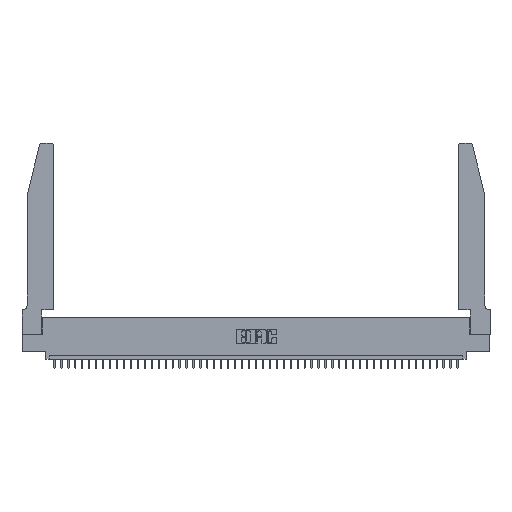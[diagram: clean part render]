
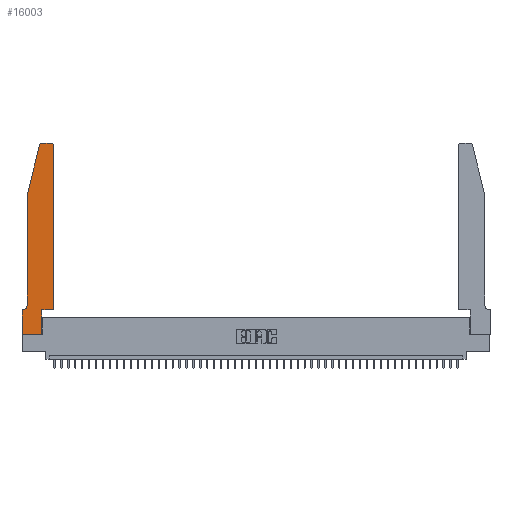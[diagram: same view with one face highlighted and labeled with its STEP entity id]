
A CAD part, top view. The second image highlights one B-rep face of the part: STEP entity #16003.
In plain terms, the highlighted planar face has unit normal (0, 0, 1).
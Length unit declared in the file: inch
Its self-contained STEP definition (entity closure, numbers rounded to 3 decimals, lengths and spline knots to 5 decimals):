
#1456 = AXIS2_PLACEMENT_3D ( 'NONE', #13694, #27518, #30842 ) ;
#2073 = VECTOR ( 'NONE', #4219, 39.37008 ) ;
#2291 = VERTEX_POINT ( 'NONE', #4777 ) ;
#2474 = ORIENTED_EDGE ( 'NONE', *, *, #27144, .T. ) ;
#3057 = CIRCLE ( 'NONE', #18257, 0.07 ) ;
#3388 = LINE ( 'NONE', #43634, #18350 ) ;
#4219 = DIRECTION ( 'NONE',  ( 0., 1., 0. ) ) ;
#4227 = CARTESIAN_POINT ( 'NONE',  ( 0., 0., 0.37 ) ) ;
#4251 = EDGE_CURVE ( 'NONE', #35111, #40724, #8358, .T. ) ;
#4667 = ORIENTED_EDGE ( 'NONE', *, *, #15329, .T. ) ;
#4777 = CARTESIAN_POINT ( 'NONE',  ( 0.0055, 0.35, 0.37 ) ) ;
#4821 = CIRCLE ( 'NONE', #31468, 0.03 ) ;
#4933 = LINE ( 'NONE', #8534, #8687 ) ;
#6106 = VECTOR ( 'NONE', #23300, 39.37008 ) ;
#6298 = PLANE ( 'NONE',  #1456 ) ;
#6853 = EDGE_CURVE ( 'NONE', #2291, #31830, #31171, .T. ) ;
#6995 = ORIENTED_EDGE ( 'NONE', *, *, #8389, .T. ) ;
#7415 = DIRECTION ( 'NONE',  ( 0., 1., 0. ) ) ;
#8043 = DIRECTION ( 'NONE',  ( -0.239, -0.971, 0. ) ) ;
#8358 = CIRCLE ( 'NONE', #34991, 0.03 ) ;
#8389 = EDGE_CURVE ( 'NONE', #27132, #35111, #39346, .T. ) ;
#8534 = CARTESIAN_POINT ( 'NONE',  ( 0.0755, 2., 0.37 ) ) ;
#8687 = VECTOR ( 'NONE', #8043, 39.37008 ) ;
#8797 = DIRECTION ( 'NONE',  ( -1., 0., 0. ) ) ;
#11934 = CARTESIAN_POINT ( 'NONE',  ( 0.4205, 2.72, 0.37 ) ) ;
#12011 = VECTOR ( 'NONE', #40225, 39.37008 ) ;
#12864 = ORIENTED_EDGE ( 'NONE', *, *, #18434, .T. ) ;
#13694 = CARTESIAN_POINT ( 'NONE',  ( 0., 0.35, 0.37 ) ) ;
#13732 = EDGE_LOOP ( 'NONE', ( #6995, #37165, #42310, #45712, #12864, #44758, #30821, #14931, #4667, #2474, #36168, #24620 ) ) ;
#13870 = DIRECTION ( 'NONE',  ( -1., 0., 0. ) ) ;
#14038 = CARTESIAN_POINT ( 'NONE',  ( 0.4505, 0.35, 0.37 ) ) ;
#14585 = CARTESIAN_POINT ( 'NONE',  ( 0.4505, 2.72, 0.37 ) ) ;
#14931 = ORIENTED_EDGE ( 'NONE', *, *, #23414, .T. ) ;
#15329 = EDGE_CURVE ( 'NONE', #28963, #21868, #15487, .T. ) ;
#15487 = LINE ( 'NONE', #25520, #23508 ) ;
#16003 = ADVANCED_FACE ( 'NONE', ( #34897 ), #6298, .T. ) ;
#17102 = EDGE_CURVE ( 'NONE', #32184, #42963, #20414, .T. ) ;
#17620 = DIRECTION ( 'NONE',  ( 1., 0., 0. ) ) ;
#18257 = AXIS2_PLACEMENT_3D ( 'NONE', #24459, #38998, #38522 ) ;
#18306 = LINE ( 'NONE', #14038, #42040 ) ;
#18350 = VECTOR ( 'NONE', #25315, 39.37008 ) ;
#18434 = EDGE_CURVE ( 'NONE', #42963, #2291, #3057, .T. ) ;
#20414 = LINE ( 'NONE', #34956, #6106 ) ;
#20868 = VECTOR ( 'NONE', #13870, 39.37008 ) ;
#21611 = DIRECTION ( 'NONE',  ( 1., 0., 0. ) ) ;
#21777 = CARTESIAN_POINT ( 'NONE',  ( 0.2865, 0.35, 0.37 ) ) ;
#21868 = VERTEX_POINT ( 'NONE', #21777 ) ;
#23216 = VERTEX_POINT ( 'NONE', #40831 ) ;
#23300 = DIRECTION ( 'NONE',  ( 0., -1., 0. ) ) ;
#23414 = EDGE_CURVE ( 'NONE', #23216, #28963, #3388, .T. ) ;
#23508 = VECTOR ( 'NONE', #7415, 39.37008 ) ;
#24068 = CARTESIAN_POINT ( 'NONE',  ( 0., 0.35, 0.37 ) ) ;
#24459 = CARTESIAN_POINT ( 'NONE',  ( 0.0055, 0.42, 0.37 ) ) ;
#24620 = ORIENTED_EDGE ( 'NONE', *, *, #28134, .T. ) ;
#25315 = DIRECTION ( 'NONE',  ( 1., 0., 0. ) ) ;
#25520 = CARTESIAN_POINT ( 'NONE',  ( 0.2865, 0.35, 0.37 ) ) ;
#25915 = LINE ( 'NONE', #40457, #2073 ) ;
#26722 = VECTOR ( 'NONE', #8797, 39.37008 ) ;
#27132 = VERTEX_POINT ( 'NONE', #28329 ) ;
#27144 = EDGE_CURVE ( 'NONE', #21868, #39072, #18306, .T. ) ;
#27518 = DIRECTION ( 'NONE',  ( 0., 0., 1. ) ) ;
#28134 = EDGE_CURVE ( 'NONE', #31577, #27132, #4821, .T. ) ;
#28329 = CARTESIAN_POINT ( 'NONE',  ( 0.4205, 2.75, 0.37 ) ) ;
#28490 = EDGE_CURVE ( 'NONE', #40724, #32184, #4933, .T. ) ;
#28778 = CARTESIAN_POINT ( 'NONE',  ( 0.284, 2.72, 0.37 ) ) ;
#28963 = VERTEX_POINT ( 'NONE', #37058 ) ;
#30821 = ORIENTED_EDGE ( 'NONE', *, *, #40504, .T. ) ;
#30842 = DIRECTION ( 'NONE',  ( 1., 0., 0. ) ) ;
#31171 = LINE ( 'NONE', #45709, #26722 ) ;
#31468 = AXIS2_PLACEMENT_3D ( 'NONE', #11934, #45503, #46437 ) ;
#31577 = VERTEX_POINT ( 'NONE', #14585 ) ;
#31830 = VERTEX_POINT ( 'NONE', #24068 ) ;
#32184 = VERTEX_POINT ( 'NONE', #33559 ) ;
#32814 = DIRECTION ( 'NONE',  ( 0., 0., 1. ) ) ;
#33559 = CARTESIAN_POINT ( 'NONE',  ( 0.0755, 2., 0.37 ) ) ;
#34897 = FACE_OUTER_BOUND ( 'NONE', #13732, .T. ) ;
#34956 = CARTESIAN_POINT ( 'NONE',  ( 0.0755, 2., 0.37 ) ) ;
#34991 = AXIS2_PLACEMENT_3D ( 'NONE', #28778, #32814, #21611 ) ;
#35111 = VERTEX_POINT ( 'NONE', #41304 ) ;
#36168 = ORIENTED_EDGE ( 'NONE', *, *, #39595, .T. ) ;
#37058 = CARTESIAN_POINT ( 'NONE',  ( 0.2865, 0., 0.37 ) ) ;
#37165 = ORIENTED_EDGE ( 'NONE', *, *, #4251, .T. ) ;
#37170 = CARTESIAN_POINT ( 'NONE',  ( 0.4505, 0.35, 0.37 ) ) ;
#38522 = DIRECTION ( 'NONE',  ( -1., 0., 0. ) ) ;
#38998 = DIRECTION ( 'NONE',  ( 0., 0., -1. ) ) ;
#39072 = VERTEX_POINT ( 'NONE', #37170 ) ;
#39346 = LINE ( 'NONE', #39569, #20868 ) ;
#39569 = CARTESIAN_POINT ( 'NONE',  ( 0.2605, 2.75, 0.37 ) ) ;
#39595 = EDGE_CURVE ( 'NONE', #39072, #31577, #25915, .T. ) ;
#40225 = DIRECTION ( 'NONE',  ( 0., -1., 0. ) ) ;
#40457 = CARTESIAN_POINT ( 'NONE',  ( 0.4505, 0.35, 0.37 ) ) ;
#40504 = EDGE_CURVE ( 'NONE', #31830, #23216, #43786, .T. ) ;
#40724 = VERTEX_POINT ( 'NONE', #41866 ) ;
#40831 = CARTESIAN_POINT ( 'NONE',  ( 0., 0., 0.37 ) ) ;
#41304 = CARTESIAN_POINT ( 'NONE',  ( 0.284, 2.75, 0.37 ) ) ;
#41866 = CARTESIAN_POINT ( 'NONE',  ( 0.25487, 2.72718, 0.37 ) ) ;
#42040 = VECTOR ( 'NONE', #17620, 39.37008 ) ;
#42310 = ORIENTED_EDGE ( 'NONE', *, *, #28490, .T. ) ;
#42529 = CARTESIAN_POINT ( 'NONE',  ( 0.0755, 0.42, 0.37 ) ) ;
#42963 = VERTEX_POINT ( 'NONE', #42529 ) ;
#43634 = CARTESIAN_POINT ( 'NONE',  ( 0., 0., 0.37 ) ) ;
#43786 = LINE ( 'NONE', #4227, #12011 ) ;
#44758 = ORIENTED_EDGE ( 'NONE', *, *, #6853, .T. ) ;
#45503 = DIRECTION ( 'NONE',  ( 0., 0., 1. ) ) ;
#45709 = CARTESIAN_POINT ( 'NONE',  ( 0.0755, 0.35, 0.37 ) ) ;
#45712 = ORIENTED_EDGE ( 'NONE', *, *, #17102, .T. ) ;
#46437 = DIRECTION ( 'NONE',  ( 1., 0., 0. ) ) ;
